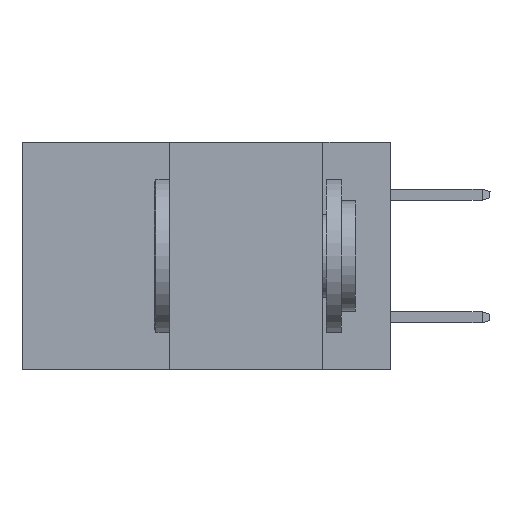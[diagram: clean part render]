
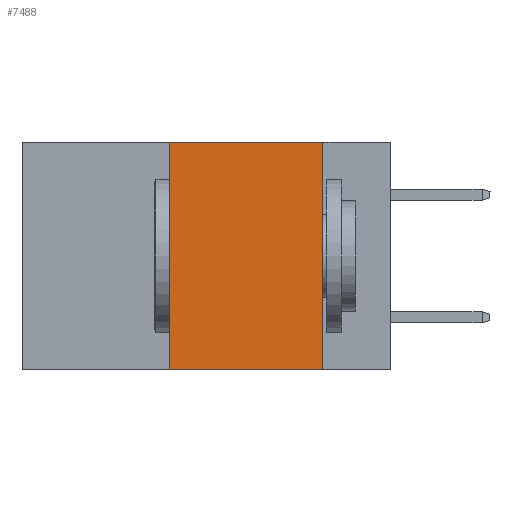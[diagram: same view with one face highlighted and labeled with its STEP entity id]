
A CAD part, left-side view. The second image highlights one B-rep face of the part: STEP entity #7488.
In plain terms, the highlighted planar face has unit normal (-1, 0, 0).
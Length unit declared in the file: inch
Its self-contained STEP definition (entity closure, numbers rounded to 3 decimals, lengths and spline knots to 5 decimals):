
#35 = CARTESIAN_POINT ( 'NONE',  ( 0., 0.11, 0. ) ) ;
#831 = PLANE ( 'NONE',  #7002 ) ;
#1574 = LINE ( 'NONE', #13484, #7617 ) ;
#1890 = DIRECTION ( 'NONE',  ( 0., -1., 0. ) ) ;
#1930 = CARTESIAN_POINT ( 'NONE',  ( 0., 0.6, -0.37 ) ) ;
#2641 = EDGE_CURVE ( 'NONE', #9521, #24217, #3778, .T. ) ;
#2941 = DIRECTION ( 'NONE',  ( 1., 0., 0. ) ) ;
#3778 = LINE ( 'NONE', #1930, #14710 ) ;
#4053 = FACE_OUTER_BOUND ( 'NONE', #16454, .T. ) ;
#7002 = AXIS2_PLACEMENT_3D ( 'NONE', #14626, #2941, #16534 ) ;
#7400 = CARTESIAN_POINT ( 'NONE',  ( 0., 0.11, 0. ) ) ;
#7488 = ADVANCED_FACE ( 'NONE', ( #4053 ), #831, .F. ) ;
#7602 = ORIENTED_EDGE ( 'NONE', *, *, #2641, .T. ) ;
#7617 = VECTOR ( 'NONE', #25018, 39.37008 ) ;
#8526 = VERTEX_POINT ( 'NONE', #35 ) ;
#9521 = VERTEX_POINT ( 'NONE', #18701 ) ;
#11257 = EDGE_CURVE ( 'NONE', #8526, #24217, #14654, .T. ) ;
#11512 = ORIENTED_EDGE ( 'NONE', *, *, #17769, .F. ) ;
#11806 = ORIENTED_EDGE ( 'NONE', *, *, #11257, .F. ) ;
#13025 = CARTESIAN_POINT ( 'NONE',  ( 0., 0.36, 0. ) ) ;
#13139 = CARTESIAN_POINT ( 'NONE',  ( 0., 0.11, -0.37 ) ) ;
#13484 = CARTESIAN_POINT ( 'NONE',  ( 0., 0.6, 0. ) ) ;
#14626 = CARTESIAN_POINT ( 'NONE',  ( 0., 0.6, 0. ) ) ;
#14654 = LINE ( 'NONE', #7400, #24296 ) ;
#14710 = VECTOR ( 'NONE', #1890, 39.37008 ) ;
#14855 = DIRECTION ( 'NONE',  ( 0., 0., 1. ) ) ;
#16454 = EDGE_LOOP ( 'NONE', ( #11806, #11512, #22295, #7602 ) ) ;
#16534 = DIRECTION ( 'NONE',  ( 0., 0., -1. ) ) ;
#17769 = EDGE_CURVE ( 'NONE', #21288, #8526, #1574, .T. ) ;
#18649 = CARTESIAN_POINT ( 'NONE',  ( 0., 0.36, 0. ) ) ;
#18701 = CARTESIAN_POINT ( 'NONE',  ( 0., 0.36, -0.37 ) ) ;
#20816 = DIRECTION ( 'NONE',  ( 0., 0., -1. ) ) ;
#21288 = VERTEX_POINT ( 'NONE', #18649 ) ;
#22295 = ORIENTED_EDGE ( 'NONE', *, *, #22955, .F. ) ;
#22955 = EDGE_CURVE ( 'NONE', #9521, #21288, #23593, .T. ) ;
#23593 = LINE ( 'NONE', #13025, #24193 ) ;
#24193 = VECTOR ( 'NONE', #14855, 39.37008 ) ;
#24217 = VERTEX_POINT ( 'NONE', #13139 ) ;
#24296 = VECTOR ( 'NONE', #20816, 39.37008 ) ;
#25018 = DIRECTION ( 'NONE',  ( 0., -1., 0. ) ) ;
